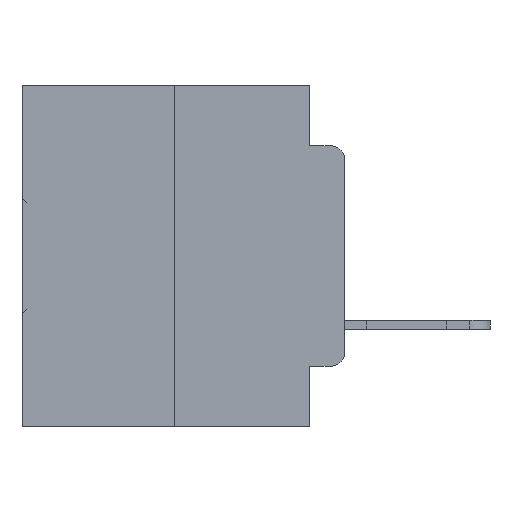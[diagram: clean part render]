
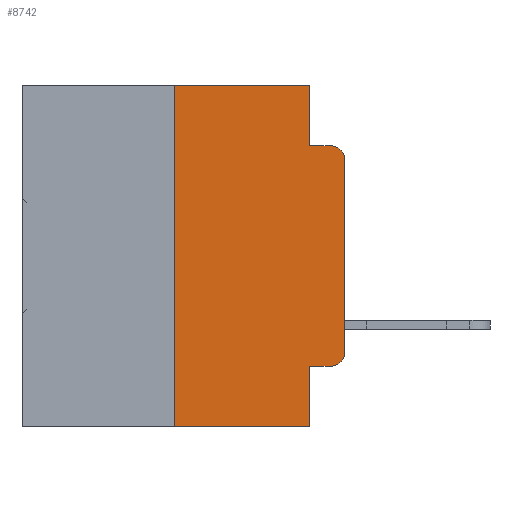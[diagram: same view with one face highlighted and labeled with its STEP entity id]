
A CAD part, left-side view. The second image highlights one B-rep face of the part: STEP entity #8742.
In plain terms, the highlighted planar face has unit normal (-1, 0, 0).
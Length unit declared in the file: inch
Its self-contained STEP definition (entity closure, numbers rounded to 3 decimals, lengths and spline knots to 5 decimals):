
#70 = CARTESIAN_POINT ( 'NONE',  ( 0., 0.25, 0. ) ) ;
#855 = EDGE_CURVE ( 'NONE', #2066, #10476, #30538, .T. ) ;
#1254 = EDGE_CURVE ( 'NONE', #10476, #5969, #3354, .T. ) ;
#1785 = EDGE_CURVE ( 'NONE', #26570, #18964, #21636, .T. ) ;
#2066 = VERTEX_POINT ( 'NONE', #70 ) ;
#2397 = VERTEX_POINT ( 'NONE', #26799 ) ;
#2433 = CARTESIAN_POINT ( 'NONE',  ( 0., 0.051, -0.4115 ) ) ;
#2561 = CARTESIAN_POINT ( 'NONE',  ( 0., 0.25, -0.5 ) ) ;
#2910 = LINE ( 'NONE', #14310, #30143 ) ;
#3354 = LINE ( 'NONE', #14466, #30509 ) ;
#3808 = AXIS2_PLACEMENT_3D ( 'NONE', #5004, #23841, #7841 ) ;
#5004 = CARTESIAN_POINT ( 'NONE',  ( 0., 0.02, -0.1085 ) ) ;
#5265 = CIRCLE ( 'NONE', #11300, 0.02 ) ;
#5467 = ORIENTED_EDGE ( 'NONE', *, *, #16680, .T. ) ;
#5969 = VERTEX_POINT ( 'NONE', #24654 ) ;
#5987 = CARTESIAN_POINT ( 'NONE',  ( 0., 0.473, 0. ) ) ;
#6725 = VERTEX_POINT ( 'NONE', #28736 ) ;
#6899 = VERTEX_POINT ( 'NONE', #2433 ) ;
#7771 = CARTESIAN_POINT ( 'NONE',  ( 0., 0.473, -0.5 ) ) ;
#7841 = DIRECTION ( 'NONE',  ( 0., 0., -1. ) ) ;
#8172 = VECTOR ( 'NONE', #32020, 39.37008 ) ;
#8313 = ORIENTED_EDGE ( 'NONE', *, *, #9354, .F. ) ;
#8668 = EDGE_CURVE ( 'NONE', #25308, #2397, #5265, .T. ) ;
#8742 = ADVANCED_FACE ( 'NONE', ( #10060 ), #18463, .F. ) ;
#9354 = EDGE_CURVE ( 'NONE', #6899, #18964, #30220, .T. ) ;
#9768 = CARTESIAN_POINT ( 'NONE',  ( 0., 0.051, -0.0885 ) ) ;
#10060 = FACE_OUTER_BOUND ( 'NONE', #11200, .T. ) ;
#10377 = DIRECTION ( 'NONE',  ( 0., 0., -1. ) ) ;
#10476 = VERTEX_POINT ( 'NONE', #13366 ) ;
#11200 = EDGE_LOOP ( 'NONE', ( #27657, #29542, #29569, #31984, #32626, #33282, #15949, #8313, #5467, #17396 ) ) ;
#11270 = DIRECTION ( 'NONE',  ( 0., -1., 0. ) ) ;
#11300 = AXIS2_PLACEMENT_3D ( 'NONE', #30652, #15545, #33028 ) ;
#12232 = VECTOR ( 'NONE', #12533, 39.37008 ) ;
#12237 = LINE ( 'NONE', #24472, #31770 ) ;
#12533 = DIRECTION ( 'NONE',  ( 0., -1., 0. ) ) ;
#13366 = CARTESIAN_POINT ( 'NONE',  ( 0., 0.051, 0. ) ) ;
#14310 = CARTESIAN_POINT ( 'NONE',  ( 0., 0., 0. ) ) ;
#14466 = CARTESIAN_POINT ( 'NONE',  ( 0., 0.051, 0. ) ) ;
#14503 = DIRECTION ( 'NONE',  ( 0., 0., -1. ) ) ;
#15478 = LINE ( 'NONE', #31917, #8172 ) ;
#15545 = DIRECTION ( 'NONE',  ( -1., 0., 0. ) ) ;
#15808 = EDGE_CURVE ( 'NONE', #6725, #29446, #24709, .T. ) ;
#15949 = ORIENTED_EDGE ( 'NONE', *, *, #1785, .T. ) ;
#15968 = DIRECTION ( 'NONE',  ( 0., -1., 0. ) ) ;
#16680 = EDGE_CURVE ( 'NONE', #6899, #25308, #12237, .T. ) ;
#16849 = VECTOR ( 'NONE', #21363, 39.37008 ) ;
#17017 = DIRECTION ( 'NONE',  ( 0., 0., 1. ) ) ;
#17215 = VECTOR ( 'NONE', #32829, 39.37008 ) ;
#17396 = ORIENTED_EDGE ( 'NONE', *, *, #8668, .T. ) ;
#18033 = CARTESIAN_POINT ( 'NONE',  ( 0., 0.02, -0.0885 ) ) ;
#18463 = PLANE ( 'NONE',  #23743 ) ;
#18769 = CARTESIAN_POINT ( 'NONE',  ( 0., 0.051, 0. ) ) ;
#18964 = VERTEX_POINT ( 'NONE', #28772 ) ;
#21299 = EDGE_CURVE ( 'NONE', #5969, #29446, #32514, .T. ) ;
#21363 = DIRECTION ( 'NONE',  ( 0., 0., -1. ) ) ;
#21510 = CARTESIAN_POINT ( 'NONE',  ( 0., 0.02, -0.4115 ) ) ;
#21636 = LINE ( 'NONE', #7771, #33781 ) ;
#23338 = EDGE_CURVE ( 'NONE', #2397, #6725, #2910, .T. ) ;
#23743 = AXIS2_PLACEMENT_3D ( 'NONE', #26059, #26155, #10377 ) ;
#23841 = DIRECTION ( 'NONE',  ( -1., 0., 0. ) ) ;
#24472 = CARTESIAN_POINT ( 'NONE',  ( 0., 0.051, -0.4115 ) ) ;
#24654 = CARTESIAN_POINT ( 'NONE',  ( 0., 0.051, -0.0885 ) ) ;
#24709 = CIRCLE ( 'NONE', #3808, 0.02 ) ;
#25308 = VERTEX_POINT ( 'NONE', #21510 ) ;
#26059 = CARTESIAN_POINT ( 'NONE',  ( 0., 0.473, 0. ) ) ;
#26155 = DIRECTION ( 'NONE',  ( 1., 0., 0. ) ) ;
#26570 = VERTEX_POINT ( 'NONE', #2561 ) ;
#26799 = CARTESIAN_POINT ( 'NONE',  ( 0., 0., -0.3915 ) ) ;
#27657 = ORIENTED_EDGE ( 'NONE', *, *, #23338, .T. ) ;
#28736 = CARTESIAN_POINT ( 'NONE',  ( 0., 0., -0.1085 ) ) ;
#28772 = CARTESIAN_POINT ( 'NONE',  ( 0., 0.051, -0.5 ) ) ;
#29165 = EDGE_CURVE ( 'NONE', #26570, #2066, #15478, .T. ) ;
#29446 = VERTEX_POINT ( 'NONE', #18033 ) ;
#29542 = ORIENTED_EDGE ( 'NONE', *, *, #15808, .T. ) ;
#29569 = ORIENTED_EDGE ( 'NONE', *, *, #21299, .F. ) ;
#30143 = VECTOR ( 'NONE', #17017, 39.37008 ) ;
#30220 = LINE ( 'NONE', #18769, #16849 ) ;
#30509 = VECTOR ( 'NONE', #14503, 39.37008 ) ;
#30538 = LINE ( 'NONE', #5987, #17215 ) ;
#30652 = CARTESIAN_POINT ( 'NONE',  ( 0., 0.02, -0.3915 ) ) ;
#31770 = VECTOR ( 'NONE', #11270, 39.37008 ) ;
#31917 = CARTESIAN_POINT ( 'NONE',  ( 0., 0.25, 0. ) ) ;
#31984 = ORIENTED_EDGE ( 'NONE', *, *, #1254, .F. ) ;
#32020 = DIRECTION ( 'NONE',  ( 0., 0., 1. ) ) ;
#32514 = LINE ( 'NONE', #9768, #12232 ) ;
#32626 = ORIENTED_EDGE ( 'NONE', *, *, #855, .F. ) ;
#32829 = DIRECTION ( 'NONE',  ( 0., -1., 0. ) ) ;
#33028 = DIRECTION ( 'NONE',  ( 0., 0., -1. ) ) ;
#33282 = ORIENTED_EDGE ( 'NONE', *, *, #29165, .F. ) ;
#33781 = VECTOR ( 'NONE', #15968, 39.37008 ) ;
